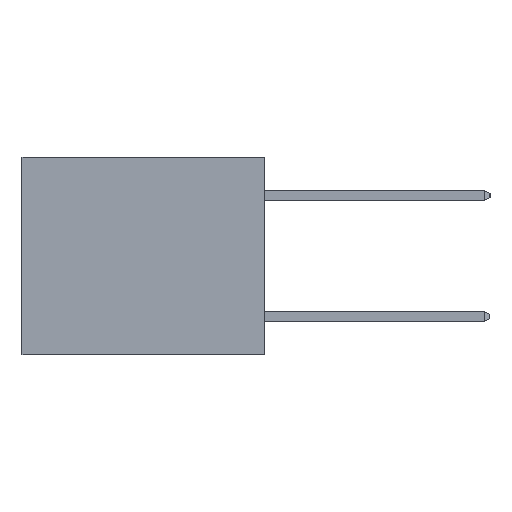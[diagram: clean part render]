
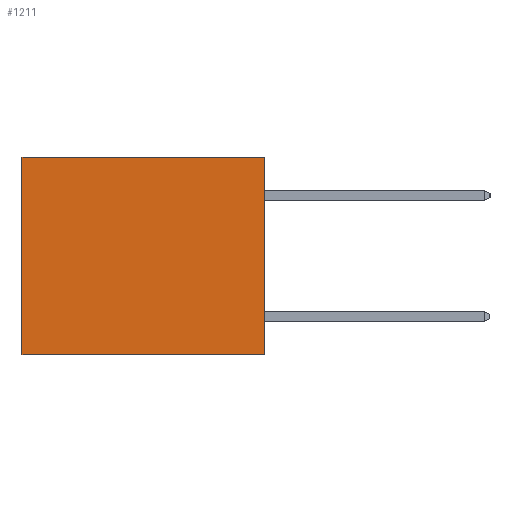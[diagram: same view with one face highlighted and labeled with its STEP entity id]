
A CAD part, left-side view. The second image highlights one B-rep face of the part: STEP entity #1211.
In plain terms, the highlighted planar face has unit normal (-1, 0, 0).
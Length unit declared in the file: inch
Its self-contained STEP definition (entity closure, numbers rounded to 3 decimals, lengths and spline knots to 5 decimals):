
#468 = LINE ( 'NONE', #8283, #17675 ) ;
#914 = LINE ( 'NONE', #2078, #17680 ) ;
#1139 = CARTESIAN_POINT ( 'NONE',  ( 0.3165, 0.6, -0.49 ) ) ;
#1211 = ADVANCED_FACE ( 'NONE', ( #15804 ), #16374, .F. ) ;
#1338 = VERTEX_POINT ( 'NONE', #5440 ) ;
#1579 = ORIENTED_EDGE ( 'NONE', *, *, #16677, .T. ) ;
#2078 = CARTESIAN_POINT ( 'NONE',  ( 0.3165, 0., -0.49 ) ) ;
#2539 = DIRECTION ( 'NONE',  ( 0., 0., -1. ) ) ;
#3203 = LINE ( 'NONE', #4503, #17593 ) ;
#3597 = VERTEX_POINT ( 'NONE', #4934 ) ;
#4503 = CARTESIAN_POINT ( 'NONE',  ( 0.3165, 0., -0.49 ) ) ;
#4689 = AXIS2_PLACEMENT_3D ( 'NONE', #15070, #12338, #8133 ) ;
#4934 = CARTESIAN_POINT ( 'NONE',  ( 0.3165, 0.6, -0.49 ) ) ;
#5196 = ORIENTED_EDGE ( 'NONE', *, *, #16852, .F. ) ;
#5440 = CARTESIAN_POINT ( 'NONE',  ( 0.3165, 0., -0.49 ) ) ;
#7566 = VECTOR ( 'NONE', #2539, 39.37008 ) ;
#8133 = DIRECTION ( 'NONE',  ( 0., 0., -1. ) ) ;
#8283 = CARTESIAN_POINT ( 'NONE',  ( 0.3165, 0., 0. ) ) ;
#8615 = VERTEX_POINT ( 'NONE', #13358 ) ;
#8694 = DIRECTION ( 'NONE',  ( 0., 1., 0. ) ) ;
#10446 = EDGE_CURVE ( 'NONE', #12729, #1338, #914, .T. ) ;
#10648 = ORIENTED_EDGE ( 'NONE', *, *, #14741, .T. ) ;
#11696 = LINE ( 'NONE', #1139, #7566 ) ;
#12338 = DIRECTION ( 'NONE',  ( 1., 0., 0. ) ) ;
#12533 = DIRECTION ( 'NONE',  ( 0., 1., 0. ) ) ;
#12729 = VERTEX_POINT ( 'NONE', #16522 ) ;
#13301 = EDGE_LOOP ( 'NONE', ( #1579, #5196, #14199, #10648 ) ) ;
#13358 = CARTESIAN_POINT ( 'NONE',  ( 0.3165, 0.6, 0. ) ) ;
#14199 = ORIENTED_EDGE ( 'NONE', *, *, #10446, .F. ) ;
#14741 = EDGE_CURVE ( 'NONE', #12729, #8615, #468, .T. ) ;
#15070 = CARTESIAN_POINT ( 'NONE',  ( 0.3165, 0., -0.49 ) ) ;
#15804 = FACE_OUTER_BOUND ( 'NONE', #13301, .T. ) ;
#16055 = DIRECTION ( 'NONE',  ( 0., 0., -1. ) ) ;
#16374 = PLANE ( 'NONE',  #4689 ) ;
#16522 = CARTESIAN_POINT ( 'NONE',  ( 0.3165, 0., 0. ) ) ;
#16677 = EDGE_CURVE ( 'NONE', #8615, #3597, #11696, .T. ) ;
#16852 = EDGE_CURVE ( 'NONE', #1338, #3597, #3203, .T. ) ;
#17593 = VECTOR ( 'NONE', #8694, 39.37008 ) ;
#17675 = VECTOR ( 'NONE', #12533, 39.37008 ) ;
#17680 = VECTOR ( 'NONE', #16055, 39.37008 ) ;
